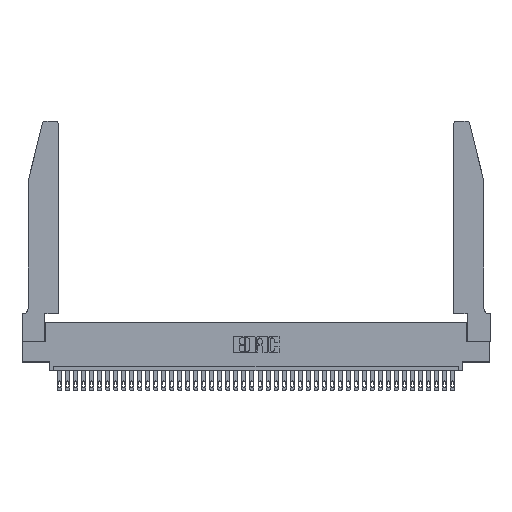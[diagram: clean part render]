
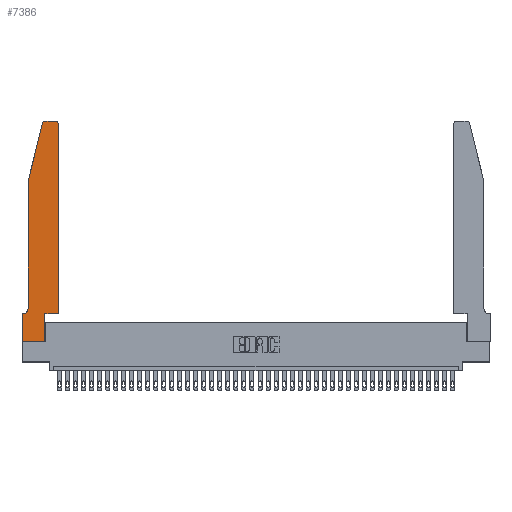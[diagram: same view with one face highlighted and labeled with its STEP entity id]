
A CAD part, top view. The second image highlights one B-rep face of the part: STEP entity #7386.
In plain terms, the highlighted planar face has unit normal (0, 0, 1).
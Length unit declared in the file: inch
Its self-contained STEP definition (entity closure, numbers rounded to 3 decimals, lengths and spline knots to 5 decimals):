
#193 = VECTOR ( 'NONE', #36824, 39.37008 ) ;
#736 = EDGE_CURVE ( 'NONE', #4595, #10260, #3187, .T. ) ;
#1894 = CARTESIAN_POINT ( 'NONE',  ( 0.25487, 2.72718, 0.37 ) ) ;
#2399 = VECTOR ( 'NONE', #23540, 39.37008 ) ;
#2499 = CARTESIAN_POINT ( 'NONE',  ( 0., 0.35, 0.37 ) ) ;
#3089 = ORIENTED_EDGE ( 'NONE', *, *, #6064, .T. ) ;
#3187 = LINE ( 'NONE', #37192, #30652 ) ;
#3463 = VERTEX_POINT ( 'NONE', #13273 ) ;
#3732 = CIRCLE ( 'NONE', #29259, 0.03 ) ;
#3945 = CARTESIAN_POINT ( 'NONE',  ( 0.0755, 2., 0.37 ) ) ;
#4389 = EDGE_LOOP ( 'NONE', ( #33402, #25612, #15574, #3089, #16792, #18753, #39766, #37713, #9077, #25519, #9566, #40518 ) ) ;
#4421 = DIRECTION ( 'NONE',  ( 1., 0., 0. ) ) ;
#4595 = VERTEX_POINT ( 'NONE', #25560 ) ;
#5163 = PLANE ( 'NONE',  #39481 ) ;
#6064 = EDGE_CURVE ( 'NONE', #38294, #24598, #10830, .T. ) ;
#6870 = DIRECTION ( 'NONE',  ( 0., 0., 1. ) ) ;
#6984 = EDGE_CURVE ( 'NONE', #20369, #3463, #36735, .T. ) ;
#7129 = VECTOR ( 'NONE', #4421, 39.37008 ) ;
#7386 = ADVANCED_FACE ( 'NONE', ( #41240 ), #5163, .T. ) ;
#7468 = EDGE_CURVE ( 'NONE', #10260, #21765, #26145, .T. ) ;
#7510 = DIRECTION ( 'NONE',  ( -1., 0., 0. ) ) ;
#8067 = EDGE_CURVE ( 'NONE', #34949, #20369, #19632, .T. ) ;
#8148 = CARTESIAN_POINT ( 'NONE',  ( 0.284, 2.72, 0.37 ) ) ;
#9077 = ORIENTED_EDGE ( 'NONE', *, *, #6984, .T. ) ;
#9143 = CARTESIAN_POINT ( 'NONE',  ( 0.4505, 0.35, 0.37 ) ) ;
#9286 = CARTESIAN_POINT ( 'NONE',  ( 0., 0., 0.37 ) ) ;
#9566 = ORIENTED_EDGE ( 'NONE', *, *, #736, .T. ) ;
#10198 = VERTEX_POINT ( 'NONE', #18257 ) ;
#10260 = VERTEX_POINT ( 'NONE', #38272 ) ;
#10661 = AXIS2_PLACEMENT_3D ( 'NONE', #35704, #26610, #7510 ) ;
#10664 = VECTOR ( 'NONE', #30237, 39.37008 ) ;
#10830 = LINE ( 'NONE', #3945, #2399 ) ;
#10835 = EDGE_CURVE ( 'NONE', #28769, #38294, #39035, .T. ) ;
#11514 = DIRECTION ( 'NONE',  ( 0., 0., 1. ) ) ;
#11600 = VECTOR ( 'NONE', #25625, 39.37008 ) ;
#11801 = VECTOR ( 'NONE', #21213, 39.37008 ) ;
#13273 = CARTESIAN_POINT ( 'NONE',  ( 0.2865, 0.35, 0.37 ) ) ;
#13994 = CARTESIAN_POINT ( 'NONE',  ( 0.0755, 2., 0.37 ) ) ;
#14469 = CARTESIAN_POINT ( 'NONE',  ( 0.2605, 2.75, 0.37 ) ) ;
#14838 = CARTESIAN_POINT ( 'NONE',  ( 0., 0., 0.37 ) ) ;
#15574 = ORIENTED_EDGE ( 'NONE', *, *, #10835, .T. ) ;
#16792 = ORIENTED_EDGE ( 'NONE', *, *, #32172, .T. ) ;
#17152 = LINE ( 'NONE', #14469, #193 ) ;
#17497 = CARTESIAN_POINT ( 'NONE',  ( 0.4205, 2.75, 0.37 ) ) ;
#18025 = DIRECTION ( 'NONE',  ( 1., 0., 0. ) ) ;
#18246 = LINE ( 'NONE', #23463, #10664 ) ;
#18257 = CARTESIAN_POINT ( 'NONE',  ( 0.0055, 0.35, 0.37 ) ) ;
#18303 = CARTESIAN_POINT ( 'NONE',  ( 0., 0.35, 0.37 ) ) ;
#18753 = ORIENTED_EDGE ( 'NONE', *, *, #35121, .T. ) ;
#19224 = CARTESIAN_POINT ( 'NONE',  ( 0.0755, 2., 0.37 ) ) ;
#19632 = LINE ( 'NONE', #14838, #7129 ) ;
#19940 = VECTOR ( 'NONE', #34505, 39.37008 ) ;
#20369 = VERTEX_POINT ( 'NONE', #24365 ) ;
#20787 = CARTESIAN_POINT ( 'NONE',  ( 0.2865, 0.35, 0.37 ) ) ;
#21213 = DIRECTION ( 'NONE',  ( 0., 1., 0. ) ) ;
#21765 = VERTEX_POINT ( 'NONE', #17497 ) ;
#22276 = VERTEX_POINT ( 'NONE', #38627 ) ;
#23302 = EDGE_CURVE ( 'NONE', #36135, #34949, #28292, .T. ) ;
#23463 = CARTESIAN_POINT ( 'NONE',  ( 0.0755, 0.35, 0.37 ) ) ;
#23540 = DIRECTION ( 'NONE',  ( 0., -1., 0. ) ) ;
#24365 = CARTESIAN_POINT ( 'NONE',  ( 0.2865, 0., 0.37 ) ) ;
#24598 = VERTEX_POINT ( 'NONE', #26869 ) ;
#24746 = EDGE_CURVE ( 'NONE', #21765, #22276, #17152, .T. ) ;
#25519 = ORIENTED_EDGE ( 'NONE', *, *, #31992, .T. ) ;
#25560 = CARTESIAN_POINT ( 'NONE',  ( 0.4505, 0.35, 0.37 ) ) ;
#25612 = ORIENTED_EDGE ( 'NONE', *, *, #34161, .T. ) ;
#25625 = DIRECTION ( 'NONE',  ( -0.239, -0.971, 0. ) ) ;
#26145 = CIRCLE ( 'NONE', #31536, 0.03 ) ;
#26167 = CARTESIAN_POINT ( 'NONE',  ( 0., 0., 0.37 ) ) ;
#26610 = DIRECTION ( 'NONE',  ( 0., 0., -1. ) ) ;
#26730 = VECTOR ( 'NONE', #41094, 39.37008 ) ;
#26869 = CARTESIAN_POINT ( 'NONE',  ( 0.0755, 0.42, 0.37 ) ) ;
#27493 = LINE ( 'NONE', #9143, #19940 ) ;
#27670 = DIRECTION ( 'NONE',  ( 0., 0., 1. ) ) ;
#27692 = DIRECTION ( 'NONE',  ( 0., 1., 0. ) ) ;
#28292 = LINE ( 'NONE', #9286, #26730 ) ;
#28769 = VERTEX_POINT ( 'NONE', #1894 ) ;
#28941 = CARTESIAN_POINT ( 'NONE',  ( 0.4205, 2.72, 0.37 ) ) ;
#29259 = AXIS2_PLACEMENT_3D ( 'NONE', #8148, #11514, #37054 ) ;
#30237 = DIRECTION ( 'NONE',  ( -1., 0., 0. ) ) ;
#30652 = VECTOR ( 'NONE', #27692, 39.37008 ) ;
#31536 = AXIS2_PLACEMENT_3D ( 'NONE', #28941, #6870, #35343 ) ;
#31992 = EDGE_CURVE ( 'NONE', #3463, #4595, #27493, .T. ) ;
#32172 = EDGE_CURVE ( 'NONE', #24598, #10198, #39919, .T. ) ;
#33402 = ORIENTED_EDGE ( 'NONE', *, *, #24746, .T. ) ;
#34161 = EDGE_CURVE ( 'NONE', #22276, #28769, #3732, .T. ) ;
#34505 = DIRECTION ( 'NONE',  ( 1., 0., 0. ) ) ;
#34949 = VERTEX_POINT ( 'NONE', #26167 ) ;
#35121 = EDGE_CURVE ( 'NONE', #10198, #36135, #18246, .T. ) ;
#35343 = DIRECTION ( 'NONE',  ( 1., 0., 0. ) ) ;
#35704 = CARTESIAN_POINT ( 'NONE',  ( 0.0055, 0.42, 0.37 ) ) ;
#36135 = VERTEX_POINT ( 'NONE', #2499 ) ;
#36735 = LINE ( 'NONE', #20787, #11801 ) ;
#36824 = DIRECTION ( 'NONE',  ( -1., 0., 0. ) ) ;
#37054 = DIRECTION ( 'NONE',  ( 1., 0., 0. ) ) ;
#37192 = CARTESIAN_POINT ( 'NONE',  ( 0.4505, 0.35, 0.37 ) ) ;
#37713 = ORIENTED_EDGE ( 'NONE', *, *, #8067, .T. ) ;
#38272 = CARTESIAN_POINT ( 'NONE',  ( 0.4505, 2.72, 0.37 ) ) ;
#38294 = VERTEX_POINT ( 'NONE', #13994 ) ;
#38627 = CARTESIAN_POINT ( 'NONE',  ( 0.284, 2.75, 0.37 ) ) ;
#39035 = LINE ( 'NONE', #19224, #11600 ) ;
#39481 = AXIS2_PLACEMENT_3D ( 'NONE', #18303, #27670, #18025 ) ;
#39766 = ORIENTED_EDGE ( 'NONE', *, *, #23302, .T. ) ;
#39919 = CIRCLE ( 'NONE', #10661, 0.07 ) ;
#40518 = ORIENTED_EDGE ( 'NONE', *, *, #7468, .T. ) ;
#41094 = DIRECTION ( 'NONE',  ( 0., -1., 0. ) ) ;
#41240 = FACE_OUTER_BOUND ( 'NONE', #4389, .T. ) ;
